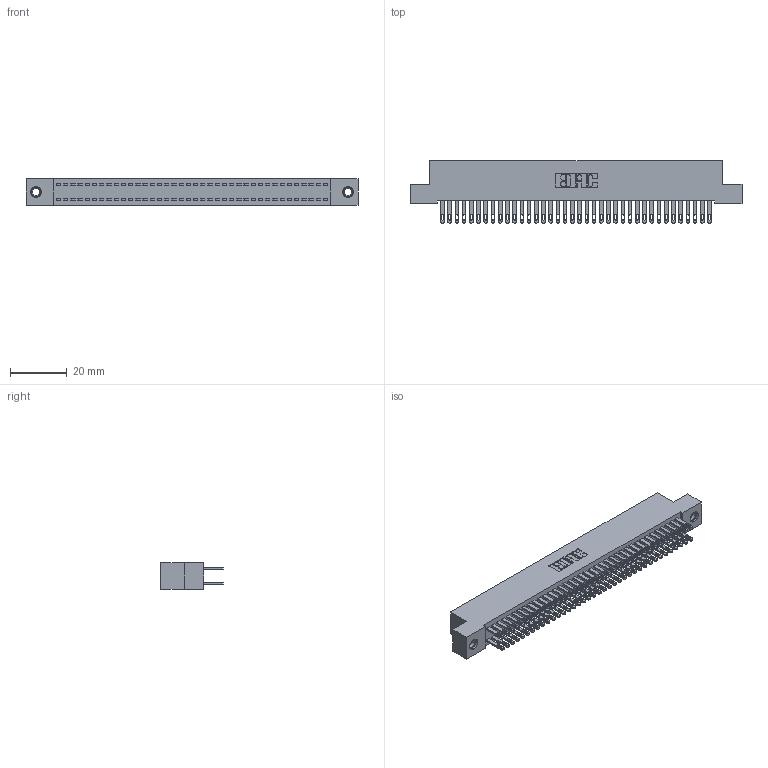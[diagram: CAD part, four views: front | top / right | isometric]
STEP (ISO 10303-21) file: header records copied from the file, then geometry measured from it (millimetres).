
FILE_DESCRIPTION (( 'STEP AP203' ), '1' );
FILE_NAME ('342-076-500-207.STEP', '2018-08-13T12:03:04', ( '' ), ( '' ), 'SwSTEP 2.0', 'SolidWorks 2016', '' );
FILE_SCHEMA (( 'CONFIG_CONTROL_DESIGN' ));
Length unit declared in the file: inch
Products named in the file (4): 345-292-001_345-293-100; 345-250-001_345-250-005-103; 342-076-500-207; 342 Part_TI
Assembly tree (79 placements, depth 2):
  342-076-500-207
    342 Part_TI
    345-292-001_345-293-100  x76
    345-250-001_345-250-005-103  x2
Bounding box: 116.84 x 21.85 x 9.4 mm (x, y, z)
Volume: 10698.7 mm3; surface area: 18069.6 mm2
Topology: 79 solids, 79 shells, 3818 faces, 11607 edges, 7730 vertices
Faces by surface type: plane 2378, cylinder 1424, cone 12, torus 4
Entity records: 25948 total; most frequent: CARTESIAN_POINT 4285, ORIENTED_EDGE 4214, DIRECTION 3701, EDGE_CURVE 2107, VECTOR 1955, LINE 1955, VERTEX_POINT 1400, AXIS2_PLACEMENT_3D 873
